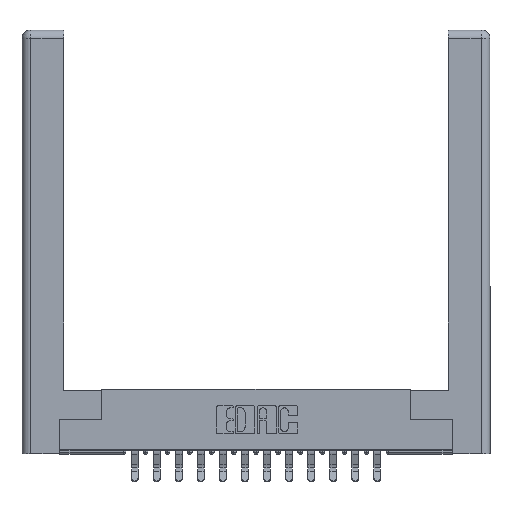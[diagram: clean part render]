
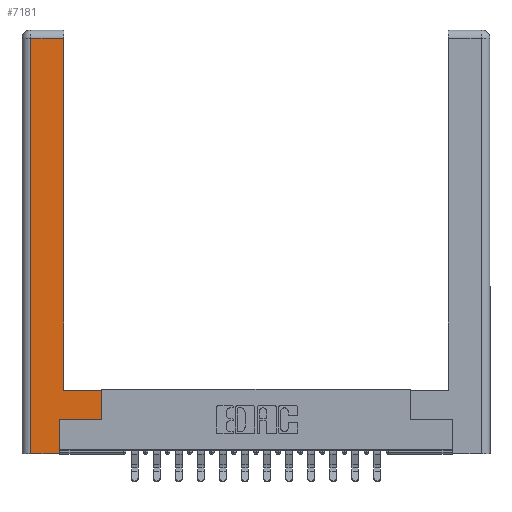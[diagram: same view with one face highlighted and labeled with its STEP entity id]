
A CAD part, top view. The second image highlights one B-rep face of the part: STEP entity #7181.
In plain terms, the highlighted planar face has unit normal (0, 0, 1).
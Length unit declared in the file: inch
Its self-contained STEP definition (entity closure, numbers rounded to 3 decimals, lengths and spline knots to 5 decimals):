
#147 = VERTEX_POINT ( 'NONE', #18010 ) ;
#333 = CARTESIAN_POINT ( 'NONE',  ( 0.565, 0.45, 0. ) ) ;
#732 = FACE_OUTER_BOUND ( 'NONE', #1564, .T. ) ;
#812 = VECTOR ( 'NONE', #6881, 39.37008 ) ;
#941 = CARTESIAN_POINT ( 'NONE',  ( 0.565, 0.245, 0. ) ) ;
#991 = ORIENTED_EDGE ( 'NONE', *, *, #15609, .T. ) ;
#1564 = EDGE_LOOP ( 'NONE', ( #17167, #1643, #991, #6206, #7508, #1571, #14065, #13752 ) ) ;
#1571 = ORIENTED_EDGE ( 'NONE', *, *, #4961, .T. ) ;
#1643 = ORIENTED_EDGE ( 'NONE', *, *, #14208, .T. ) ;
#1856 = CARTESIAN_POINT ( 'NONE',  ( 0.0615, 0., 0. ) ) ;
#2388 = VERTEX_POINT ( 'NONE', #17439 ) ;
#2796 = VERTEX_POINT ( 'NONE', #18739 ) ;
#3308 = AXIS2_PLACEMENT_3D ( 'NONE', #15757, #8276, #5232 ) ;
#3374 = EDGE_CURVE ( 'NONE', #13853, #147, #10750, .T. ) ;
#3599 = LINE ( 'NONE', #10684, #15597 ) ;
#3850 = VERTEX_POINT ( 'NONE', #18304 ) ;
#4071 = DIRECTION ( 'NONE',  ( 1., 0., 0. ) ) ;
#4961 = EDGE_CURVE ( 'NONE', #11381, #5339, #11843, .T. ) ;
#5021 = DIRECTION ( 'NONE',  ( 1., 0., 0. ) ) ;
#5056 = VECTOR ( 'NONE', #5021, 39.37008 ) ;
#5232 = DIRECTION ( 'NONE',  ( -1., 0., 0. ) ) ;
#5339 = VERTEX_POINT ( 'NONE', #13668 ) ;
#5399 = VECTOR ( 'NONE', #6493, 39.37008 ) ;
#5481 = DIRECTION ( 'NONE',  ( 0., 1., 0. ) ) ;
#6193 = EDGE_CURVE ( 'NONE', #5339, #13853, #3599, .T. ) ;
#6206 = ORIENTED_EDGE ( 'NONE', *, *, #15157, .T. ) ;
#6493 = DIRECTION ( 'NONE',  ( -1., 0., 0. ) ) ;
#6839 = CARTESIAN_POINT ( 'NONE',  ( 0.295, 0.45, 0. ) ) ;
#6881 = DIRECTION ( 'NONE',  ( 0., 1., 0. ) ) ;
#7181 = ADVANCED_FACE ( 'NONE', ( #732 ), #12731, .F. ) ;
#7508 = ORIENTED_EDGE ( 'NONE', *, *, #11181, .T. ) ;
#7670 = LINE ( 'NONE', #8270, #812 ) ;
#7885 = VECTOR ( 'NONE', #4071, 39.37008 ) ;
#8087 = CARTESIAN_POINT ( 'NONE',  ( 0.0615, 2.94, 0. ) ) ;
#8121 = VECTOR ( 'NONE', #10801, 39.37008 ) ;
#8167 = VECTOR ( 'NONE', #5481, 39.37008 ) ;
#8270 = CARTESIAN_POINT ( 'NONE',  ( 0.295, 3., 0. ) ) ;
#8276 = DIRECTION ( 'NONE',  ( 0., 0., -1. ) ) ;
#9576 = CARTESIAN_POINT ( 'NONE',  ( 0.265, 0.245, 0. ) ) ;
#10257 = LINE ( 'NONE', #14042, #5056 ) ;
#10684 = CARTESIAN_POINT ( 'NONE',  ( 0.565, 0.45, 0. ) ) ;
#10750 = LINE ( 'NONE', #6839, #19470 ) ;
#10801 = DIRECTION ( 'NONE',  ( 0., -1., 0. ) ) ;
#11181 = EDGE_CURVE ( 'NONE', #17055, #11381, #13098, .T. ) ;
#11381 = VERTEX_POINT ( 'NONE', #16457 ) ;
#11843 = LINE ( 'NONE', #941, #7885 ) ;
#12464 = CARTESIAN_POINT ( 'NONE',  ( 0.265, 0., 0. ) ) ;
#12731 = PLANE ( 'NONE',  #3308 ) ;
#13098 = LINE ( 'NONE', #9576, #8167 ) ;
#13515 = LINE ( 'NONE', #1856, #8121 ) ;
#13627 = LINE ( 'NONE', #8087, #5399 ) ;
#13668 = CARTESIAN_POINT ( 'NONE',  ( 0.565, 0.245, 0. ) ) ;
#13752 = ORIENTED_EDGE ( 'NONE', *, *, #3374, .T. ) ;
#13853 = VERTEX_POINT ( 'NONE', #333 ) ;
#14042 = CARTESIAN_POINT ( 'NONE',  ( 0.265, 0., 0. ) ) ;
#14065 = ORIENTED_EDGE ( 'NONE', *, *, #6193, .T. ) ;
#14208 = EDGE_CURVE ( 'NONE', #2388, #3850, #13627, .T. ) ;
#15157 = EDGE_CURVE ( 'NONE', #2796, #17055, #10257, .T. ) ;
#15287 = EDGE_CURVE ( 'NONE', #147, #2388, #7670, .T. ) ;
#15568 = DIRECTION ( 'NONE',  ( -1., 0., 0. ) ) ;
#15597 = VECTOR ( 'NONE', #18172, 39.37008 ) ;
#15609 = EDGE_CURVE ( 'NONE', #3850, #2796, #13515, .T. ) ;
#15757 = CARTESIAN_POINT ( 'NONE',  ( 0., 0., 0. ) ) ;
#16457 = CARTESIAN_POINT ( 'NONE',  ( 0.265, 0.245, 0. ) ) ;
#17055 = VERTEX_POINT ( 'NONE', #12464 ) ;
#17167 = ORIENTED_EDGE ( 'NONE', *, *, #15287, .T. ) ;
#17439 = CARTESIAN_POINT ( 'NONE',  ( 0.295, 2.94, 0. ) ) ;
#18010 = CARTESIAN_POINT ( 'NONE',  ( 0.295, 0.45, 0. ) ) ;
#18172 = DIRECTION ( 'NONE',  ( 0., 1., 0. ) ) ;
#18304 = CARTESIAN_POINT ( 'NONE',  ( 0.0615, 2.94, 0. ) ) ;
#18739 = CARTESIAN_POINT ( 'NONE',  ( 0.0615, 0., 0. ) ) ;
#19470 = VECTOR ( 'NONE', #15568, 39.37008 ) ;
